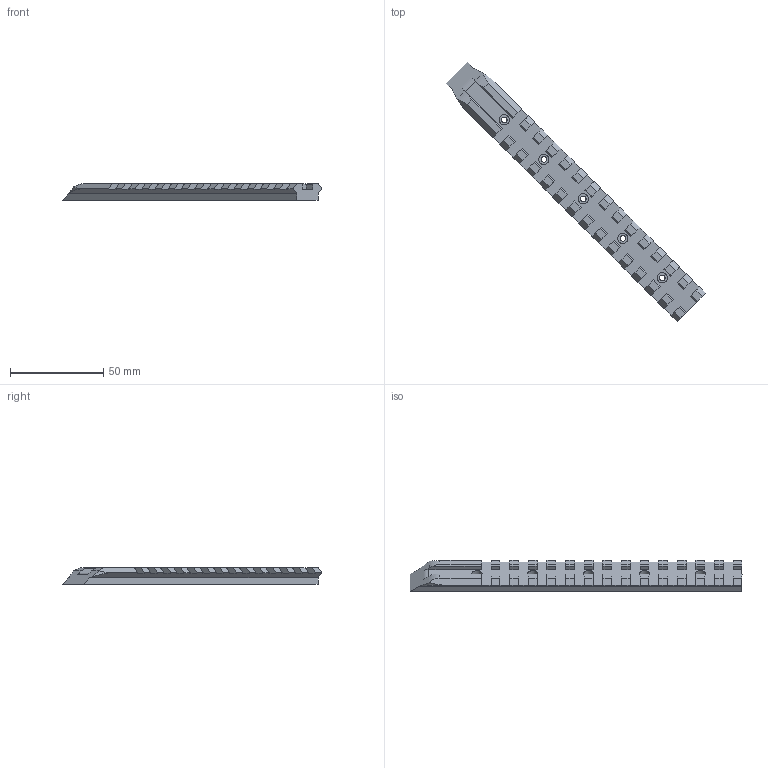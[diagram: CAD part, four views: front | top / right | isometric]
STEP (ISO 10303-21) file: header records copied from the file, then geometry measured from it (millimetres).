
FILE_DESCRIPTION(/* description */ (''),/* implementation_level */ '2;1');
FILE_NAME(/* name */ 'Top Rail Back Half.step',/* time_stamp */ '2022-05-11T21:21:49-06:00',/* author */ (''),/* organization */ (''),/* preprocessor_version */ 'ST-DEVELOPER v18.1',/* originating_system */ 'Autodesk Translation Framework v10.10.0.1391',/* authorisation */ '');
FILE_SCHEMA (('AUTOMOTIVE_DESIGN { 1 0 10303 214 3 1 1 }'));
Length unit declared in the file: millimetre
Products named in the file (1): Top Rail tall back (1)
Bounding box: 139.45 x 139.45 x 9 mm (x, y, z)
Volume: 20576.2 mm3; surface area: 11407.3 mm2
Topology: 1 solids, 1 shells, 206 faces, 595 edges, 396 vertices
Faces by surface type: plane 191, cylinder 15
Full cylindrical faces by diameter (mm): 3 x5, 5.5 x5
Entity records: 6721 total; most frequent: CARTESIAN_POINT 1204, ORIENTED_EDGE 1190, DIRECTION 1043, EDGE_CURVE 595, LINE 557, VECTOR 557, VERTEX_POINT 396, AXIS2_PLACEMENT_3D 243
